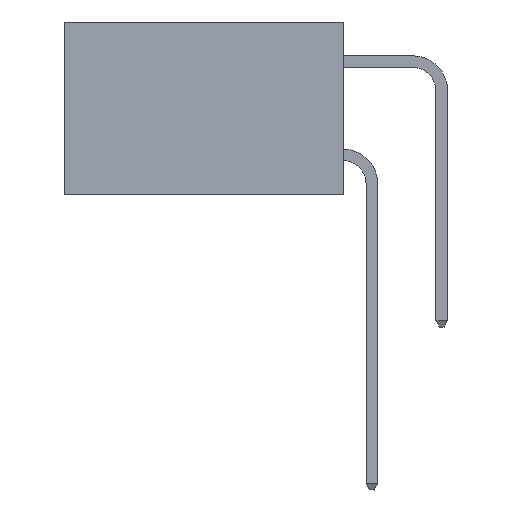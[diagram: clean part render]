
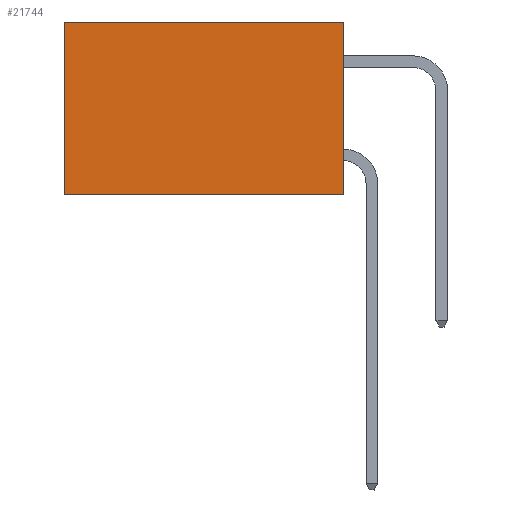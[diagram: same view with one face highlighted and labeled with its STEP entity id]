
A CAD part, left-side view. The second image highlights one B-rep face of the part: STEP entity #21744.
In plain terms, the highlighted planar face has unit normal (-1, 0, 0).
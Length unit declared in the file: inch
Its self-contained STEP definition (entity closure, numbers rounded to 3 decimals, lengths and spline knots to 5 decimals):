
#466 = ORIENTED_EDGE ( 'NONE', *, *, #23616, .T. ) ;
#1486 = CARTESIAN_POINT ( 'NONE',  ( 0.2615, 0., -0.37 ) ) ;
#1749 = VERTEX_POINT ( 'NONE', #1486 ) ;
#1875 = DIRECTION ( 'NONE',  ( 0., 0., -1. ) ) ;
#2652 = EDGE_CURVE ( 'NONE', #16125, #21181, #5943, .T. ) ;
#4077 = CARTESIAN_POINT ( 'NONE',  ( 0.2615, 0., -0.37 ) ) ;
#4175 = DIRECTION ( 'NONE',  ( 0., 1., 0. ) ) ;
#5663 = EDGE_CURVE ( 'NONE', #16125, #1749, #9016, .T. ) ;
#5943 = LINE ( 'NONE', #26579, #19203 ) ;
#6852 = AXIS2_PLACEMENT_3D ( 'NONE', #4077, #13042, #1875 ) ;
#6954 = DIRECTION ( 'NONE',  ( 0., 0., -1. ) ) ;
#8928 = PLANE ( 'NONE',  #6852 ) ;
#9016 = LINE ( 'NONE', #26852, #24640 ) ;
#9336 = VECTOR ( 'NONE', #21463, 39.37008 ) ;
#9408 = EDGE_CURVE ( 'NONE', #1749, #15582, #12453, .T. ) ;
#12453 = LINE ( 'NONE', #14077, #18263 ) ;
#13042 = DIRECTION ( 'NONE',  ( 1., 0., 0. ) ) ;
#14077 = CARTESIAN_POINT ( 'NONE',  ( 0.2615, 0., -0.37 ) ) ;
#15165 = ORIENTED_EDGE ( 'NONE', *, *, #9408, .F. ) ;
#15582 = VERTEX_POINT ( 'NONE', #15784 ) ;
#15695 = ORIENTED_EDGE ( 'NONE', *, *, #5663, .F. ) ;
#15784 = CARTESIAN_POINT ( 'NONE',  ( 0.2615, 0.6, -0.37 ) ) ;
#16125 = VERTEX_POINT ( 'NONE', #17677 ) ;
#16841 = EDGE_LOOP ( 'NONE', ( #466, #15165, #15695, #28584 ) ) ;
#17206 = LINE ( 'NONE', #19698, #9336 ) ;
#17677 = CARTESIAN_POINT ( 'NONE',  ( 0.2615, 0., 0. ) ) ;
#17950 = CARTESIAN_POINT ( 'NONE',  ( 0.2615, 0.6, 0. ) ) ;
#18263 = VECTOR ( 'NONE', #21286, 39.37008 ) ;
#19203 = VECTOR ( 'NONE', #4175, 39.37008 ) ;
#19698 = CARTESIAN_POINT ( 'NONE',  ( 0.2615, 0.6, -0.37 ) ) ;
#21181 = VERTEX_POINT ( 'NONE', #17950 ) ;
#21286 = DIRECTION ( 'NONE',  ( 0., 1., 0. ) ) ;
#21463 = DIRECTION ( 'NONE',  ( 0., 0., -1. ) ) ;
#21744 = ADVANCED_FACE ( 'NONE', ( #21890 ), #8928, .F. ) ;
#21890 = FACE_OUTER_BOUND ( 'NONE', #16841, .T. ) ;
#23616 = EDGE_CURVE ( 'NONE', #21181, #15582, #17206, .T. ) ;
#24640 = VECTOR ( 'NONE', #6954, 39.37008 ) ;
#26579 = CARTESIAN_POINT ( 'NONE',  ( 0.2615, 0., 0. ) ) ;
#26852 = CARTESIAN_POINT ( 'NONE',  ( 0.2615, 0., -0.37 ) ) ;
#28584 = ORIENTED_EDGE ( 'NONE', *, *, #2652, .T. ) ;
